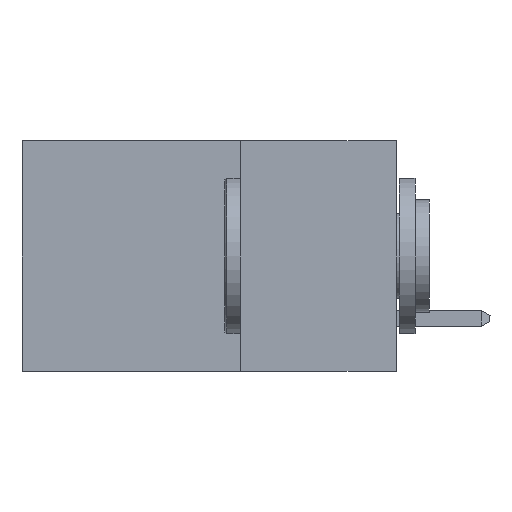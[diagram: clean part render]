
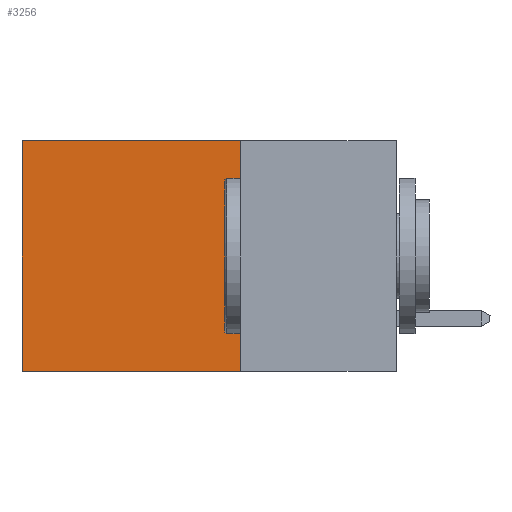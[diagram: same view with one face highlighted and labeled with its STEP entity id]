
A CAD part, left-side view. The second image highlights one B-rep face of the part: STEP entity #3256.
In plain terms, the highlighted planar face has unit normal (-1, 0, 0).
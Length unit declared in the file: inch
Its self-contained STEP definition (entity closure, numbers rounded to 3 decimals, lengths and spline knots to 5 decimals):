
#426 = CARTESIAN_POINT ( 'NONE',  ( 0.2615, 0.6, -0.37 ) ) ;
#504 = EDGE_CURVE ( 'NONE', #19269, #729, #14857, .T. ) ;
#729 = VERTEX_POINT ( 'NONE', #426 ) ;
#941 = DIRECTION ( 'NONE',  ( 0., 1., 0. ) ) ;
#1831 = ORIENTED_EDGE ( 'NONE', *, *, #504, .T. ) ;
#2200 = VECTOR ( 'NONE', #18000, 39.37008 ) ;
#3014 = LINE ( 'NONE', #9659, #11750 ) ;
#3068 = EDGE_CURVE ( 'NONE', #14650, #19269, #12467, .T. ) ;
#3256 = ADVANCED_FACE ( 'NONE', ( #13863 ), #4125, .F. ) ;
#3914 = EDGE_CURVE ( 'NONE', #14650, #4565, #19599, .T. ) ;
#4125 = PLANE ( 'NONE',  #17146 ) ;
#4503 = DIRECTION ( 'NONE',  ( 0., 1., 0. ) ) ;
#4565 = VERTEX_POINT ( 'NONE', #12349 ) ;
#4890 = EDGE_LOOP ( 'NONE', ( #1831, #8126, #5584, #15189 ) ) ;
#5557 = DIRECTION ( 'NONE',  ( 1., 0., 0. ) ) ;
#5564 = EDGE_CURVE ( 'NONE', #4565, #729, #3014, .T. ) ;
#5584 = ORIENTED_EDGE ( 'NONE', *, *, #3914, .F. ) ;
#8126 = ORIENTED_EDGE ( 'NONE', *, *, #5564, .F. ) ;
#8279 = CARTESIAN_POINT ( 'NONE',  ( 0.2615, 0.6, -0.37 ) ) ;
#9659 = CARTESIAN_POINT ( 'NONE',  ( 0.2615, 0.25, -0.37 ) ) ;
#9725 = CARTESIAN_POINT ( 'NONE',  ( 0.2615, 0.25, 0. ) ) ;
#9792 = VECTOR ( 'NONE', #4503, 39.37008 ) ;
#11750 = VECTOR ( 'NONE', #941, 39.37008 ) ;
#12246 = VECTOR ( 'NONE', #12624, 39.37008 ) ;
#12349 = CARTESIAN_POINT ( 'NONE',  ( 0.2615, 0.25, -0.37 ) ) ;
#12467 = LINE ( 'NONE', #9725, #9792 ) ;
#12624 = DIRECTION ( 'NONE',  ( 0., 0., -1. ) ) ;
#13533 = CARTESIAN_POINT ( 'NONE',  ( 0.2615, 0.6, 0. ) ) ;
#13753 = DIRECTION ( 'NONE',  ( 0., 0., -1. ) ) ;
#13863 = FACE_OUTER_BOUND ( 'NONE', #4890, .T. ) ;
#14650 = VERTEX_POINT ( 'NONE', #21316 ) ;
#14857 = LINE ( 'NONE', #8279, #2200 ) ;
#15189 = ORIENTED_EDGE ( 'NONE', *, *, #3068, .T. ) ;
#15902 = CARTESIAN_POINT ( 'NONE',  ( 0.2615, 0.25, -0.37 ) ) ;
#17146 = AXIS2_PLACEMENT_3D ( 'NONE', #18652, #5557, #13753 ) ;
#18000 = DIRECTION ( 'NONE',  ( 0., 0., -1. ) ) ;
#18652 = CARTESIAN_POINT ( 'NONE',  ( 0.2615, 0.25, -0.37 ) ) ;
#19269 = VERTEX_POINT ( 'NONE', #13533 ) ;
#19599 = LINE ( 'NONE', #15902, #12246 ) ;
#21316 = CARTESIAN_POINT ( 'NONE',  ( 0.2615, 0.25, 0. ) ) ;
